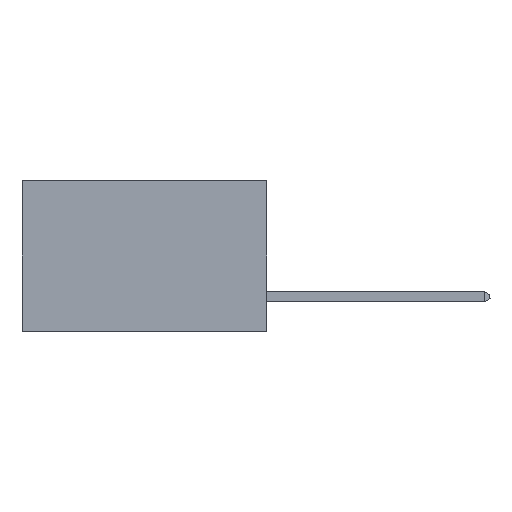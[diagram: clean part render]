
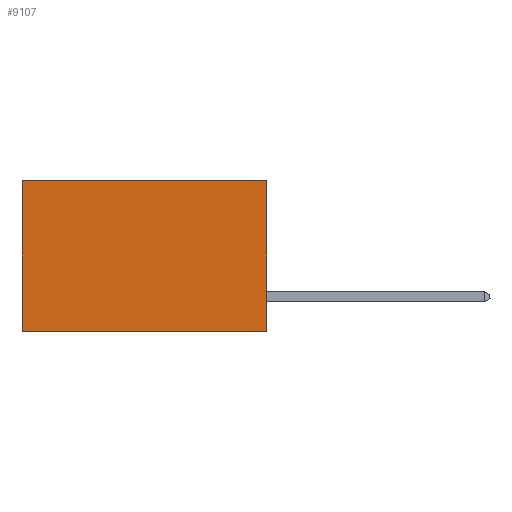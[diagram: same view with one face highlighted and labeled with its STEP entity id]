
A CAD part, left-side view. The second image highlights one B-rep face of the part: STEP entity #9107.
In plain terms, the highlighted planar face has unit normal (-1, 0, 0).
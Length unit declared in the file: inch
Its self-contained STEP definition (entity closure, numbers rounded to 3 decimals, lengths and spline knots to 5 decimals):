
#1394 = VERTEX_POINT ( 'NONE', #8549 ) ;
#2291 = DIRECTION ( 'NONE',  ( 1., 0., 0. ) ) ;
#2617 = VERTEX_POINT ( 'NONE', #13418 ) ;
#3698 = LINE ( 'NONE', #17071, #21565 ) ;
#4077 = CARTESIAN_POINT ( 'NONE',  ( 0.2875, 0., 0. ) ) ;
#5294 = DIRECTION ( 'NONE',  ( 0., 0., -1. ) ) ;
#5652 = DIRECTION ( 'NONE',  ( 0., 1., 0. ) ) ;
#6898 = CARTESIAN_POINT ( 'NONE',  ( 0.2875, 0., 0. ) ) ;
#6984 = EDGE_CURVE ( 'NONE', #2617, #9234, #14272, .T. ) ;
#8154 = AXIS2_PLACEMENT_3D ( 'NONE', #6898, #2291, #18665 ) ;
#8549 = CARTESIAN_POINT ( 'NONE',  ( 0.2875, 0.6, 0. ) ) ;
#9107 = ADVANCED_FACE ( 'NONE', ( #24217 ), #30031, .F. ) ;
#9234 = VERTEX_POINT ( 'NONE', #11960 ) ;
#9253 = ORIENTED_EDGE ( 'NONE', *, *, #29031, .T. ) ;
#9877 = VECTOR ( 'NONE', #5652, 39.37008 ) ;
#11960 = CARTESIAN_POINT ( 'NONE',  ( 0.2875, 0., -0.37 ) ) ;
#13416 = ORIENTED_EDGE ( 'NONE', *, *, #6984, .F. ) ;
#13418 = CARTESIAN_POINT ( 'NONE',  ( 0.2875, 0., 0. ) ) ;
#14272 = LINE ( 'NONE', #26687, #18983 ) ;
#17071 = CARTESIAN_POINT ( 'NONE',  ( 0.2875, 0.6, 0. ) ) ;
#18355 = VERTEX_POINT ( 'NONE', #23209 ) ;
#18665 = DIRECTION ( 'NONE',  ( 0., 0., -1. ) ) ;
#18983 = VECTOR ( 'NONE', #24469, 39.37008 ) ;
#20345 = DIRECTION ( 'NONE',  ( 0., 1., 0. ) ) ;
#21565 = VECTOR ( 'NONE', #5294, 39.37008 ) ;
#21922 = ORIENTED_EDGE ( 'NONE', *, *, #25982, .F. ) ;
#22287 = LINE ( 'NONE', #26549, #9877 ) ;
#23025 = EDGE_CURVE ( 'NONE', #2617, #1394, #23194, .T. ) ;
#23194 = LINE ( 'NONE', #4077, #27850 ) ;
#23209 = CARTESIAN_POINT ( 'NONE',  ( 0.2875, 0.6, -0.37 ) ) ;
#23650 = EDGE_LOOP ( 'NONE', ( #9253, #21922, #13416, #25836 ) ) ;
#24217 = FACE_OUTER_BOUND ( 'NONE', #23650, .T. ) ;
#24469 = DIRECTION ( 'NONE',  ( 0., 0., -1. ) ) ;
#25836 = ORIENTED_EDGE ( 'NONE', *, *, #23025, .T. ) ;
#25982 = EDGE_CURVE ( 'NONE', #9234, #18355, #22287, .T. ) ;
#26549 = CARTESIAN_POINT ( 'NONE',  ( 0.2875, 0., -0.37 ) ) ;
#26687 = CARTESIAN_POINT ( 'NONE',  ( 0.2875, 0., 0. ) ) ;
#27850 = VECTOR ( 'NONE', #20345, 39.37008 ) ;
#29031 = EDGE_CURVE ( 'NONE', #1394, #18355, #3698, .T. ) ;
#30031 = PLANE ( 'NONE',  #8154 ) ;
